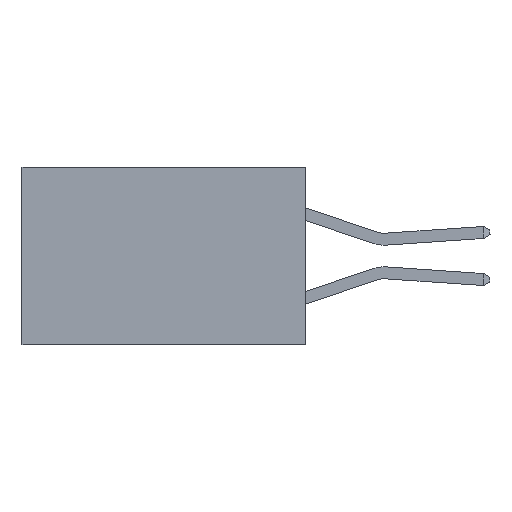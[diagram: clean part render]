
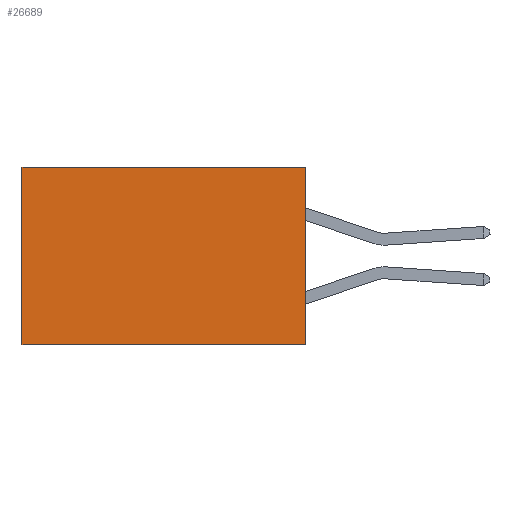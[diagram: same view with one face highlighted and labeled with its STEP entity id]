
A CAD part, left-side view. The second image highlights one B-rep face of the part: STEP entity #26689.
In plain terms, the highlighted planar face has unit normal (-1, 0, 0).
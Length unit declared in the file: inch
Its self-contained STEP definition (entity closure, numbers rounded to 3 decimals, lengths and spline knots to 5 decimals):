
#149 = VECTOR ( 'NONE', #19885, 39.37008 ) ;
#2542 = CARTESIAN_POINT ( 'NONE',  ( 0.277, 0., -0.37 ) ) ;
#3338 = EDGE_LOOP ( 'NONE', ( #25293, #24470, #9293, #17185 ) ) ;
#5487 = EDGE_CURVE ( 'NONE', #27581, #21859, #20062, .T. ) ;
#6516 = PLANE ( 'NONE',  #10075 ) ;
#6519 = DIRECTION ( 'NONE',  ( 0., 0., -1. ) ) ;
#7867 = VECTOR ( 'NONE', #11808, 39.37008 ) ;
#8567 = CARTESIAN_POINT ( 'NONE',  ( 0.277, 0., -0.37 ) ) ;
#8585 = CARTESIAN_POINT ( 'NONE',  ( 0.277, 0., 0. ) ) ;
#8664 = DIRECTION ( 'NONE',  ( 1., 0., 0. ) ) ;
#9063 = LINE ( 'NONE', #16741, #19914 ) ;
#9293 = ORIENTED_EDGE ( 'NONE', *, *, #12926, .F. ) ;
#10075 = AXIS2_PLACEMENT_3D ( 'NONE', #21619, #8664, #23770 ) ;
#10127 = EDGE_CURVE ( 'NONE', #11558, #21859, #23031, .T. ) ;
#10595 = CARTESIAN_POINT ( 'NONE',  ( 0.277, 0.59, -0.37 ) ) ;
#11558 = VERTEX_POINT ( 'NONE', #19815 ) ;
#11773 = CARTESIAN_POINT ( 'NONE',  ( 0.277, 0.59, -0.37 ) ) ;
#11808 = DIRECTION ( 'NONE',  ( 0., 0., -1. ) ) ;
#12926 = EDGE_CURVE ( 'NONE', #26084, #11558, #16485, .T. ) ;
#15081 = FACE_OUTER_BOUND ( 'NONE', #3338, .T. ) ;
#16485 = LINE ( 'NONE', #8567, #17875 ) ;
#16741 = CARTESIAN_POINT ( 'NONE',  ( 0.277, 0., 0. ) ) ;
#17185 = ORIENTED_EDGE ( 'NONE', *, *, #21755, .T. ) ;
#17875 = VECTOR ( 'NONE', #6519, 39.37008 ) ;
#19652 = CARTESIAN_POINT ( 'NONE',  ( 0.277, 0.59, 0. ) ) ;
#19815 = CARTESIAN_POINT ( 'NONE',  ( 0.277, 0., -0.37 ) ) ;
#19885 = DIRECTION ( 'NONE',  ( 0., 1., 0. ) ) ;
#19914 = VECTOR ( 'NONE', #21118, 39.37008 ) ;
#20062 = LINE ( 'NONE', #11773, #7867 ) ;
#21118 = DIRECTION ( 'NONE',  ( 0., 1., 0. ) ) ;
#21619 = CARTESIAN_POINT ( 'NONE',  ( 0.277, 0., -0.37 ) ) ;
#21755 = EDGE_CURVE ( 'NONE', #26084, #27581, #9063, .T. ) ;
#21859 = VERTEX_POINT ( 'NONE', #10595 ) ;
#23031 = LINE ( 'NONE', #2542, #149 ) ;
#23770 = DIRECTION ( 'NONE',  ( 0., 0., -1. ) ) ;
#24470 = ORIENTED_EDGE ( 'NONE', *, *, #10127, .F. ) ;
#25293 = ORIENTED_EDGE ( 'NONE', *, *, #5487, .T. ) ;
#26084 = VERTEX_POINT ( 'NONE', #8585 ) ;
#26689 = ADVANCED_FACE ( 'NONE', ( #15081 ), #6516, .F. ) ;
#27581 = VERTEX_POINT ( 'NONE', #19652 ) ;
